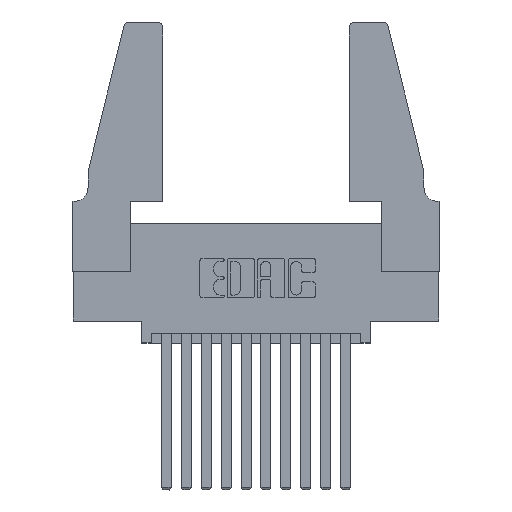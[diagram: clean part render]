
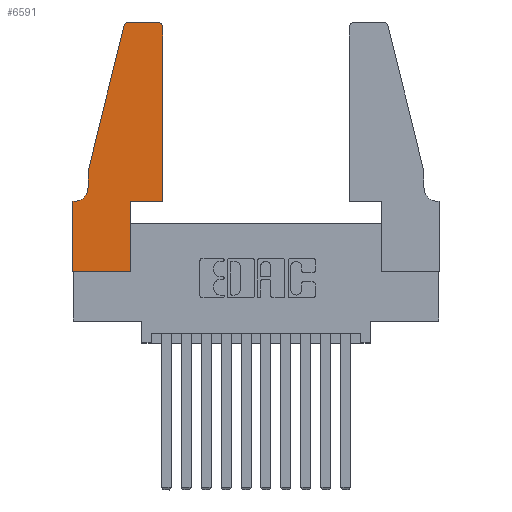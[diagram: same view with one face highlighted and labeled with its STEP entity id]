
A CAD part, top view. The second image highlights one B-rep face of the part: STEP entity #6591.
In plain terms, the highlighted planar face has unit normal (0, 0, 1).
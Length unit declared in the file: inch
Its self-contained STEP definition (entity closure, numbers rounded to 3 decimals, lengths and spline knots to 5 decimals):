
#48 = VERTEX_POINT ( 'NONE', #9750 ) ;
#329 = ORIENTED_EDGE ( 'NONE', *, *, #10738, .T. ) ;
#526 = VECTOR ( 'NONE', #1459, 39.37008 ) ;
#623 = CARTESIAN_POINT ( 'NONE',  ( 0.0755, 0.5, 0.37 ) ) ;
#778 = CIRCLE ( 'NONE', #10031, 0.07 ) ;
#1034 = CARTESIAN_POINT ( 'NONE',  ( 0.25487, 1.22718, 0.37 ) ) ;
#1272 = ORIENTED_EDGE ( 'NONE', *, *, #5073, .T. ) ;
#1273 = CARTESIAN_POINT ( 'NONE',  ( 0., 0., 0.37 ) ) ;
#1459 = DIRECTION ( 'NONE',  ( 0., -1., 0. ) ) ;
#1482 = LINE ( 'NONE', #5566, #1647 ) ;
#1629 = EDGE_CURVE ( 'NONE', #48, #13076, #778, .T. ) ;
#1647 = VECTOR ( 'NONE', #11182, 39.37008 ) ;
#1909 = DIRECTION ( 'NONE',  ( 1., 0., 0. ) ) ;
#1931 = CARTESIAN_POINT ( 'NONE',  ( 0.4505, 0.35, 0.37 ) ) ;
#2222 = CIRCLE ( 'NONE', #12501, 0.03 ) ;
#2465 = CARTESIAN_POINT ( 'NONE',  ( 0., 0., 0.37 ) ) ;
#2517 = EDGE_CURVE ( 'NONE', #7233, #8381, #4927, .T. ) ;
#2602 = EDGE_CURVE ( 'NONE', #4076, #7299, #13323, .T. ) ;
#2669 = LINE ( 'NONE', #1931, #10750 ) ;
#3031 = VECTOR ( 'NONE', #4866, 39.37008 ) ;
#3260 = EDGE_LOOP ( 'NONE', ( #3711, #6285, #329, #1272, #10986, #13061, #8688, #7099, #6908, #8111, #13581, #7801 ) ) ;
#3456 = CARTESIAN_POINT ( 'NONE',  ( 0., 0.35, 0.37 ) ) ;
#3480 = VECTOR ( 'NONE', #6546, 39.37008 ) ;
#3489 = DIRECTION ( 'NONE',  ( -1., 0., 0. ) ) ;
#3558 = EDGE_CURVE ( 'NONE', #13076, #3867, #7952, .T. ) ;
#3711 = ORIENTED_EDGE ( 'NONE', *, *, #7089, .T. ) ;
#3867 = VERTEX_POINT ( 'NONE', #6115 ) ;
#4076 = VERTEX_POINT ( 'NONE', #6258 ) ;
#4257 = VECTOR ( 'NONE', #10426, 39.37008 ) ;
#4312 = CARTESIAN_POINT ( 'NONE',  ( 0.4505, 1.22, 0.37 ) ) ;
#4357 = LINE ( 'NONE', #6626, #3480 ) ;
#4777 = LINE ( 'NONE', #9185, #4257 ) ;
#4849 = EDGE_CURVE ( 'NONE', #13072, #5486, #2222, .T. ) ;
#4866 = DIRECTION ( 'NONE',  ( -0.239, -0.971, 0. ) ) ;
#4900 = AXIS2_PLACEMENT_3D ( 'NONE', #3456, #13193, #5464 ) ;
#4909 = CARTESIAN_POINT ( 'NONE',  ( 0.284, 1.22, 0.37 ) ) ;
#4927 = CIRCLE ( 'NONE', #11662, 0.03 ) ;
#5073 = EDGE_CURVE ( 'NONE', #9672, #48, #4357, .T. ) ;
#5211 = EDGE_CURVE ( 'NONE', #13355, #7070, #6389, .T. ) ;
#5256 = VECTOR ( 'NONE', #11718, 39.37008 ) ;
#5464 = DIRECTION ( 'NONE',  ( 1., 0., 0. ) ) ;
#5486 = VERTEX_POINT ( 'NONE', #11824 ) ;
#5566 = CARTESIAN_POINT ( 'NONE',  ( 0.2605, 1.25, 0.37 ) ) ;
#5673 = DIRECTION ( 'NONE',  ( 1., 0., 0. ) ) ;
#6115 = CARTESIAN_POINT ( 'NONE',  ( 0., 0.35, 0.37 ) ) ;
#6139 = DIRECTION ( 'NONE',  ( 1., 0., 0. ) ) ;
#6258 = CARTESIAN_POINT ( 'NONE',  ( 0.2865, 0.35, 0.37 ) ) ;
#6285 = ORIENTED_EDGE ( 'NONE', *, *, #2517, .T. ) ;
#6294 = CARTESIAN_POINT ( 'NONE',  ( 0.0055, 0.42, 0.37 ) ) ;
#6389 = LINE ( 'NONE', #2465, #11905 ) ;
#6475 = CARTESIAN_POINT ( 'NONE',  ( 0.4505, 0.35, 0.37 ) ) ;
#6546 = DIRECTION ( 'NONE',  ( 0., -1., 0. ) ) ;
#6563 = PLANE ( 'NONE',  #4900 ) ;
#6591 = ADVANCED_FACE ( 'NONE', ( #7029 ), #6563, .T. ) ;
#6626 = CARTESIAN_POINT ( 'NONE',  ( 0.0755, 0.5, 0.37 ) ) ;
#6830 = CARTESIAN_POINT ( 'NONE',  ( 0., 0., 0.37 ) ) ;
#6908 = ORIENTED_EDGE ( 'NONE', *, *, #11010, .T. ) ;
#6996 = LINE ( 'NONE', #623, #3031 ) ;
#7029 = FACE_OUTER_BOUND ( 'NONE', #3260, .T. ) ;
#7070 = VERTEX_POINT ( 'NONE', #13699 ) ;
#7089 = EDGE_CURVE ( 'NONE', #5486, #7233, #1482, .T. ) ;
#7099 = ORIENTED_EDGE ( 'NONE', *, *, #5211, .T. ) ;
#7233 = VERTEX_POINT ( 'NONE', #13396 ) ;
#7299 = VERTEX_POINT ( 'NONE', #6475 ) ;
#7391 = DIRECTION ( 'NONE',  ( 0., 0., -1. ) ) ;
#7801 = ORIENTED_EDGE ( 'NONE', *, *, #4849, .T. ) ;
#7952 = LINE ( 'NONE', #13276, #9291 ) ;
#8111 = ORIENTED_EDGE ( 'NONE', *, *, #2602, .T. ) ;
#8381 = VERTEX_POINT ( 'NONE', #1034 ) ;
#8688 = ORIENTED_EDGE ( 'NONE', *, *, #12856, .T. ) ;
#9185 = CARTESIAN_POINT ( 'NONE',  ( 0.2865, 0.35, 0.37 ) ) ;
#9291 = VECTOR ( 'NONE', #3489, 39.37008 ) ;
#9388 = DIRECTION ( 'NONE',  ( 0., 0., 1. ) ) ;
#9672 = VERTEX_POINT ( 'NONE', #11895 ) ;
#9750 = CARTESIAN_POINT ( 'NONE',  ( 0.0755, 0.42, 0.37 ) ) ;
#10031 = AXIS2_PLACEMENT_3D ( 'NONE', #6294, #7391, #11933 ) ;
#10426 = DIRECTION ( 'NONE',  ( 0., 1., 0. ) ) ;
#10738 = EDGE_CURVE ( 'NONE', #8381, #9672, #6996, .T. ) ;
#10750 = VECTOR ( 'NONE', #11937, 39.37008 ) ;
#10864 = EDGE_CURVE ( 'NONE', #7299, #13072, #2669, .T. ) ;
#10986 = ORIENTED_EDGE ( 'NONE', *, *, #1629, .T. ) ;
#11010 = EDGE_CURVE ( 'NONE', #7070, #4076, #4777, .T. ) ;
#11182 = DIRECTION ( 'NONE',  ( -1., 0., 0. ) ) ;
#11662 = AXIS2_PLACEMENT_3D ( 'NONE', #4909, #12723, #6139 ) ;
#11718 = DIRECTION ( 'NONE',  ( 1., 0., 0. ) ) ;
#11824 = CARTESIAN_POINT ( 'NONE',  ( 0.4205, 1.25, 0.37 ) ) ;
#11895 = CARTESIAN_POINT ( 'NONE',  ( 0.0755, 0.5, 0.37 ) ) ;
#11905 = VECTOR ( 'NONE', #5673, 39.37008 ) ;
#11933 = DIRECTION ( 'NONE',  ( -1., 0., 0. ) ) ;
#11937 = DIRECTION ( 'NONE',  ( 0., 1., 0. ) ) ;
#12501 = AXIS2_PLACEMENT_3D ( 'NONE', #13995, #9388, #1909 ) ;
#12667 = CARTESIAN_POINT ( 'NONE',  ( 0.4505, 0.35, 0.37 ) ) ;
#12723 = DIRECTION ( 'NONE',  ( 0., 0., 1. ) ) ;
#12856 = EDGE_CURVE ( 'NONE', #3867, #13355, #13798, .T. ) ;
#13061 = ORIENTED_EDGE ( 'NONE', *, *, #3558, .T. ) ;
#13072 = VERTEX_POINT ( 'NONE', #4312 ) ;
#13076 = VERTEX_POINT ( 'NONE', #14080 ) ;
#13193 = DIRECTION ( 'NONE',  ( 0., 0., 1. ) ) ;
#13276 = CARTESIAN_POINT ( 'NONE',  ( 0.0755, 0.35, 0.37 ) ) ;
#13323 = LINE ( 'NONE', #12667, #5256 ) ;
#13355 = VERTEX_POINT ( 'NONE', #6830 ) ;
#13396 = CARTESIAN_POINT ( 'NONE',  ( 0.284, 1.25, 0.37 ) ) ;
#13581 = ORIENTED_EDGE ( 'NONE', *, *, #10864, .T. ) ;
#13699 = CARTESIAN_POINT ( 'NONE',  ( 0.2865, 0., 0.37 ) ) ;
#13798 = LINE ( 'NONE', #1273, #526 ) ;
#13995 = CARTESIAN_POINT ( 'NONE',  ( 0.4205, 1.22, 0.37 ) ) ;
#14080 = CARTESIAN_POINT ( 'NONE',  ( 0.0055, 0.35, 0.37 ) ) ;
